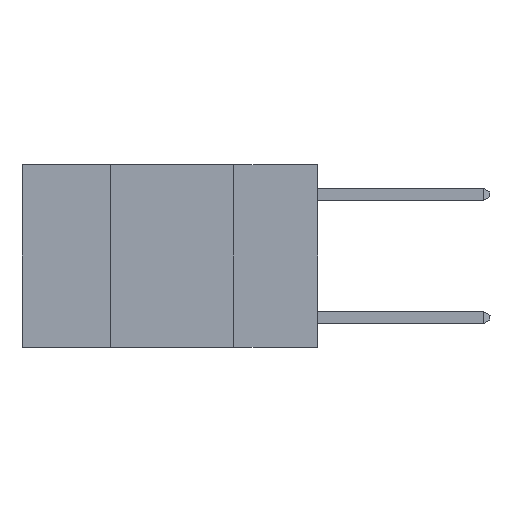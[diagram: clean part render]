
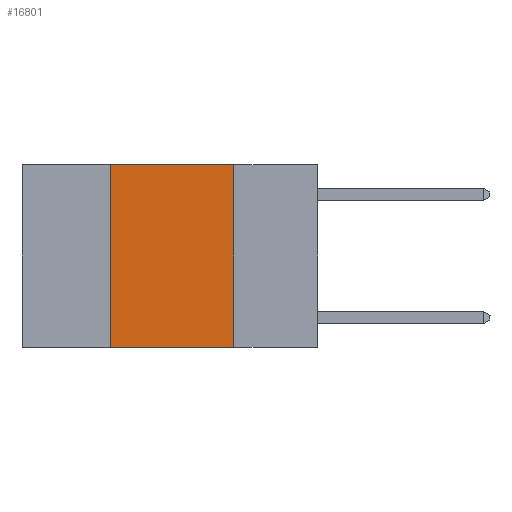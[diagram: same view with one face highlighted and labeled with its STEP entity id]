
A CAD part, left-side view. The second image highlights one B-rep face of the part: STEP entity #16801.
In plain terms, the highlighted planar face has unit normal (-1, 0, 0).
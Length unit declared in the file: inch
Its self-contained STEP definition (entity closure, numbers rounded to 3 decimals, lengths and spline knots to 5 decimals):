
#386 = EDGE_CURVE ( 'NONE', #17211, #18716, #14233, .T. ) ;
#745 = LINE ( 'NONE', #14891, #15654 ) ;
#751 = EDGE_LOOP ( 'NONE', ( #14412, #9157, #11893, #3435 ) ) ;
#1352 = CARTESIAN_POINT ( 'NONE',  ( 0., 0.6, 0. ) ) ;
#1832 = VECTOR ( 'NONE', #8675, 39.37008 ) ;
#2832 = CARTESIAN_POINT ( 'NONE',  ( 0., 0.17, 0. ) ) ;
#3435 = ORIENTED_EDGE ( 'NONE', *, *, #22916, .T. ) ;
#3992 = CARTESIAN_POINT ( 'NONE',  ( 0., 0.42, 0. ) ) ;
#4345 = AXIS2_PLACEMENT_3D ( 'NONE', #1352, #18842, #7194 ) ;
#5029 = VECTOR ( 'NONE', #7874, 39.37008 ) ;
#5203 = PLANE ( 'NONE',  #4345 ) ;
#7194 = DIRECTION ( 'NONE',  ( 0., 0., -1. ) ) ;
#7680 = EDGE_CURVE ( 'NONE', #18362, #21393, #17934, .T. ) ;
#7874 = DIRECTION ( 'NONE',  ( 0., 0., 1. ) ) ;
#8675 = DIRECTION ( 'NONE',  ( 0., 0., -1. ) ) ;
#9157 = ORIENTED_EDGE ( 'NONE', *, *, #19861, .F. ) ;
#10564 = CARTESIAN_POINT ( 'NONE',  ( 0., 0.42, 0. ) ) ;
#11604 = CARTESIAN_POINT ( 'NONE',  ( 0., 0.6, 0. ) ) ;
#11798 = CARTESIAN_POINT ( 'NONE',  ( 0., 0.17, -0.37 ) ) ;
#11893 = ORIENTED_EDGE ( 'NONE', *, *, #386, .F. ) ;
#12139 = VECTOR ( 'NONE', #21156, 39.37008 ) ;
#12232 = CARTESIAN_POINT ( 'NONE',  ( 0., 0.42, -0.37 ) ) ;
#14233 = LINE ( 'NONE', #10564, #5029 ) ;
#14412 = ORIENTED_EDGE ( 'NONE', *, *, #7680, .F. ) ;
#14891 = CARTESIAN_POINT ( 'NONE',  ( 0., 0.6, -0.37 ) ) ;
#15654 = VECTOR ( 'NONE', #16800, 39.37008 ) ;
#16800 = DIRECTION ( 'NONE',  ( 0., -1., 0. ) ) ;
#16801 = ADVANCED_FACE ( 'NONE', ( #18610 ), #5203, .F. ) ;
#17211 = VERTEX_POINT ( 'NONE', #12232 ) ;
#17881 = LINE ( 'NONE', #11604, #12139 ) ;
#17934 = LINE ( 'NONE', #2832, #1832 ) ;
#18362 = VERTEX_POINT ( 'NONE', #18534 ) ;
#18534 = CARTESIAN_POINT ( 'NONE',  ( 0., 0.17, 0. ) ) ;
#18610 = FACE_OUTER_BOUND ( 'NONE', #751, .T. ) ;
#18716 = VERTEX_POINT ( 'NONE', #3992 ) ;
#18842 = DIRECTION ( 'NONE',  ( 1., 0., 0. ) ) ;
#19861 = EDGE_CURVE ( 'NONE', #18716, #18362, #17881, .T. ) ;
#21156 = DIRECTION ( 'NONE',  ( 0., -1., 0. ) ) ;
#21393 = VERTEX_POINT ( 'NONE', #11798 ) ;
#22916 = EDGE_CURVE ( 'NONE', #17211, #21393, #745, .T. ) ;
